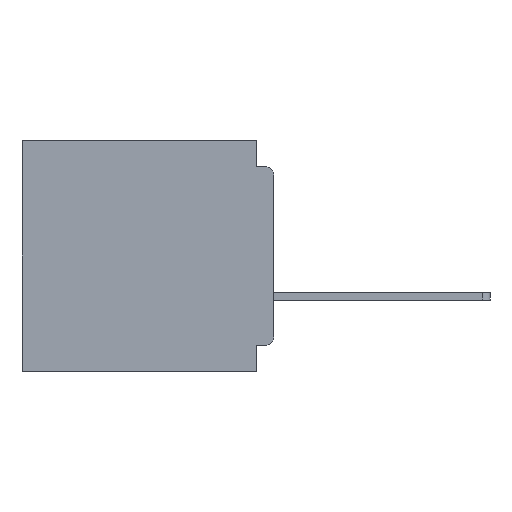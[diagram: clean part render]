
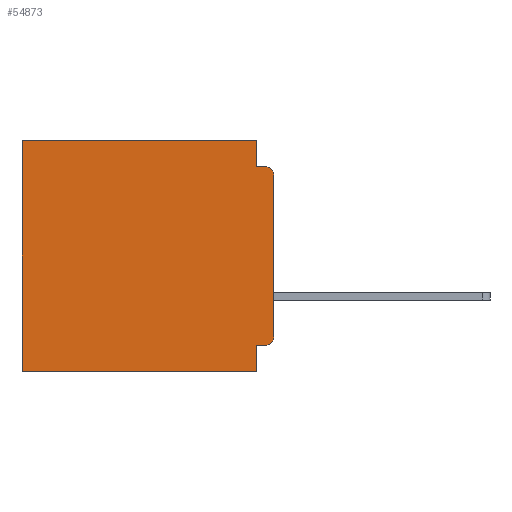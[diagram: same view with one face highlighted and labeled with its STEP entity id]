
A CAD part, left-side view. The second image highlights one B-rep face of the part: STEP entity #54873.
In plain terms, the highlighted planar face has unit normal (-1, 0, 0).
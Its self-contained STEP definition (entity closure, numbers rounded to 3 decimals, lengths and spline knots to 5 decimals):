
#1501 = VERTEX_POINT ( 'NONE', #38775 ) ;
#3084 = DIRECTION ( 'NONE',  ( 0., 0., -1. ) ) ;
#4343 = VECTOR ( 'NONE', #50784, 39.37008 ) ;
#4548 = CARTESIAN_POINT ( 'NONE',  ( 0.3, 0.437, 0. ) ) ;
#5006 = DIRECTION ( 'NONE',  ( 0., 1., 0. ) ) ;
#5340 = VERTEX_POINT ( 'NONE', #59190 ) ;
#5877 = ORIENTED_EDGE ( 'NONE', *, *, #51001, .T. ) ;
#7340 = CARTESIAN_POINT ( 'NONE',  ( 0.3, 0.015, -0.06 ) ) ;
#9245 = VERTEX_POINT ( 'NONE', #47964 ) ;
#9255 = VERTEX_POINT ( 'NONE', #4548 ) ;
#9413 = CARTESIAN_POINT ( 'NONE',  ( 0.3, 0.015, -0.34 ) ) ;
#10738 = ORIENTED_EDGE ( 'NONE', *, *, #60982, .F. ) ;
#10948 = FACE_OUTER_BOUND ( 'NONE', #27164, .T. ) ;
#12184 = DIRECTION ( 'NONE',  ( 0., 0., -1. ) ) ;
#12511 = CARTESIAN_POINT ( 'NONE',  ( 0.3, 0., -0.4 ) ) ;
#12724 = VERTEX_POINT ( 'NONE', #43125 ) ;
#12881 = VECTOR ( 'NONE', #5006, 39.37008 ) ;
#14254 = DIRECTION ( 'NONE',  ( 0., 0., -1. ) ) ;
#14826 = DIRECTION ( 'NONE',  ( 1., 0., 0. ) ) ;
#14992 = AXIS2_PLACEMENT_3D ( 'NONE', #7340, #41274, #12184 ) ;
#15619 = CARTESIAN_POINT ( 'NONE',  ( 0.3, 0.031, -0.4 ) ) ;
#16449 = CARTESIAN_POINT ( 'NONE',  ( 0.3, 0.437, -0.4 ) ) ;
#16962 = CARTESIAN_POINT ( 'NONE',  ( 0.3, 0., -0.355 ) ) ;
#18488 = CARTESIAN_POINT ( 'NONE',  ( 0.3, 0.031, -0.355 ) ) ;
#19092 = DIRECTION ( 'NONE',  ( 0., -1., 0. ) ) ;
#19175 = VERTEX_POINT ( 'NONE', #18488 ) ;
#20197 = CARTESIAN_POINT ( 'NONE',  ( 0.3, 0.437, -0.4 ) ) ;
#20349 = EDGE_CURVE ( 'NONE', #45792, #55730, #39321, .T. ) ;
#21751 = EDGE_CURVE ( 'NONE', #19175, #40889, #51860, .T. ) ;
#21869 = LINE ( 'NONE', #12511, #33283 ) ;
#23145 = VECTOR ( 'NONE', #3084, 39.37008 ) ;
#25287 = EDGE_CURVE ( 'NONE', #1501, #12724, #21869, .T. ) ;
#25666 = LINE ( 'NONE', #20197, #48351 ) ;
#26530 = CARTESIAN_POINT ( 'NONE',  ( 0.3, 0., -0.4 ) ) ;
#26627 = CIRCLE ( 'NONE', #46186, 0.015 ) ;
#27164 = EDGE_LOOP ( 'NONE', ( #62642, #32361, #10738, #35975, #29803, #48486, #61890, #43720, #55199, #5877 ) ) ;
#27195 = DIRECTION ( 'NONE',  ( 0., 0., -1. ) ) ;
#27282 = CARTESIAN_POINT ( 'NONE',  ( 0.3, 0.031, -0.4 ) ) ;
#29111 = LINE ( 'NONE', #26530, #40426 ) ;
#29577 = DIRECTION ( 'NONE',  ( 0., 0., -1. ) ) ;
#29803 = ORIENTED_EDGE ( 'NONE', *, *, #33491, .T. ) ;
#32361 = ORIENTED_EDGE ( 'NONE', *, *, #42789, .T. ) ;
#32462 = VECTOR ( 'NONE', #19092, 39.37008 ) ;
#33283 = VECTOR ( 'NONE', #27195, 39.37008 ) ;
#33491 = EDGE_CURVE ( 'NONE', #45792, #9255, #49988, .T. ) ;
#34077 = CARTESIAN_POINT ( 'NONE',  ( 0.3, 0., 0. ) ) ;
#35975 = ORIENTED_EDGE ( 'NONE', *, *, #20349, .F. ) ;
#36194 = VERTEX_POINT ( 'NONE', #16449 ) ;
#36287 = VECTOR ( 'NONE', #29577, 39.37008 ) ;
#38072 = AXIS2_PLACEMENT_3D ( 'NONE', #43865, #14826, #48709 ) ;
#38775 = CARTESIAN_POINT ( 'NONE',  ( 0.3, 0., -0.06 ) ) ;
#39070 = CARTESIAN_POINT ( 'NONE',  ( 0.3, 0.031, 0. ) ) ;
#39321 = LINE ( 'NONE', #39070, #36287 ) ;
#40395 = EDGE_CURVE ( 'NONE', #9245, #19175, #41517, .T. ) ;
#40426 = VECTOR ( 'NONE', #55428, 39.37008 ) ;
#40889 = VERTEX_POINT ( 'NONE', #15619 ) ;
#41274 = DIRECTION ( 'NONE',  ( -1., 0., 0. ) ) ;
#41517 = LINE ( 'NONE', #16962, #4343 ) ;
#42789 = EDGE_CURVE ( 'NONE', #1501, #5340, #60022, .T. ) ;
#43125 = CARTESIAN_POINT ( 'NONE',  ( 0.3, 0., -0.34 ) ) ;
#43306 = DIRECTION ( 'NONE',  ( -1., 0., 0. ) ) ;
#43720 = ORIENTED_EDGE ( 'NONE', *, *, #21751, .F. ) ;
#43865 = CARTESIAN_POINT ( 'NONE',  ( 0.3, 0., -0.4 ) ) ;
#45792 = VERTEX_POINT ( 'NONE', #62591 ) ;
#46186 = AXIS2_PLACEMENT_3D ( 'NONE', #9413, #43306, #14254 ) ;
#47964 = CARTESIAN_POINT ( 'NONE',  ( 0.3, 0.015, -0.355 ) ) ;
#48351 = VECTOR ( 'NONE', #49171, 39.37008 ) ;
#48486 = ORIENTED_EDGE ( 'NONE', *, *, #53263, .T. ) ;
#48709 = DIRECTION ( 'NONE',  ( 0., 0., -1. ) ) ;
#49171 = DIRECTION ( 'NONE',  ( 0., 0., -1. ) ) ;
#49988 = LINE ( 'NONE', #34077, #12881 ) ;
#50784 = DIRECTION ( 'NONE',  ( 0., 1., 0. ) ) ;
#51001 = EDGE_CURVE ( 'NONE', #9245, #12724, #26627, .T. ) ;
#51860 = LINE ( 'NONE', #27282, #23145 ) ;
#52884 = CARTESIAN_POINT ( 'NONE',  ( 0.3, 0., -0.045 ) ) ;
#53263 = EDGE_CURVE ( 'NONE', #9255, #36194, #25666, .T. ) ;
#54873 = ADVANCED_FACE ( 'NONE', ( #10948 ), #58171, .F. ) ;
#55199 = ORIENTED_EDGE ( 'NONE', *, *, #40395, .F. ) ;
#55428 = DIRECTION ( 'NONE',  ( 0., 1., 0. ) ) ;
#55528 = CARTESIAN_POINT ( 'NONE',  ( 0.3, 0.031, -0.045 ) ) ;
#55730 = VERTEX_POINT ( 'NONE', #55528 ) ;
#58050 = LINE ( 'NONE', #52884, #32462 ) ;
#58171 = PLANE ( 'NONE',  #38072 ) ;
#59190 = CARTESIAN_POINT ( 'NONE',  ( 0.3, 0.015, -0.045 ) ) ;
#60022 = CIRCLE ( 'NONE', #14992, 0.015 ) ;
#60982 = EDGE_CURVE ( 'NONE', #55730, #5340, #58050, .T. ) ;
#61890 = ORIENTED_EDGE ( 'NONE', *, *, #62622, .F. ) ;
#62591 = CARTESIAN_POINT ( 'NONE',  ( 0.3, 0.031, 0. ) ) ;
#62622 = EDGE_CURVE ( 'NONE', #40889, #36194, #29111, .T. ) ;
#62642 = ORIENTED_EDGE ( 'NONE', *, *, #25287, .F. ) ;
